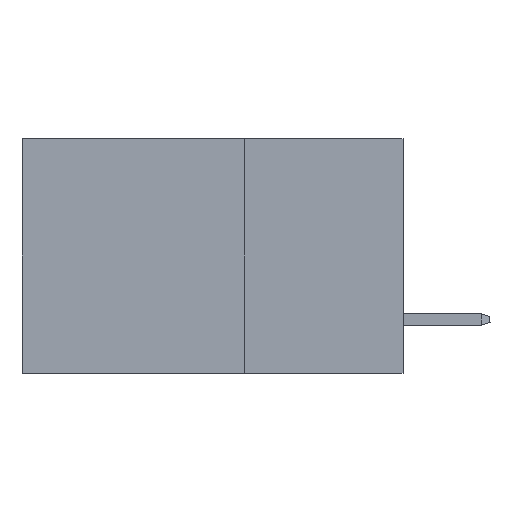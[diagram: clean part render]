
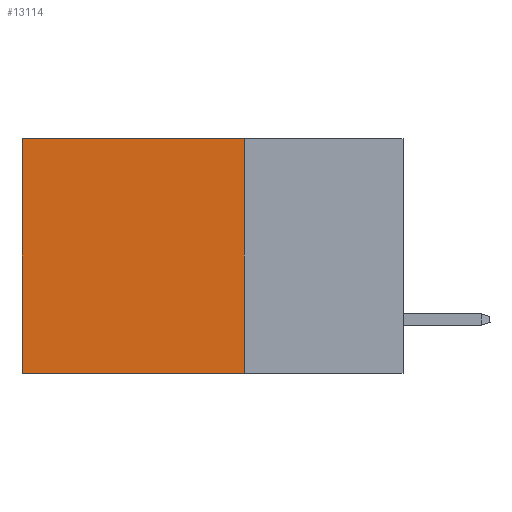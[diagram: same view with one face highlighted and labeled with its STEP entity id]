
A CAD part, left-side view. The second image highlights one B-rep face of the part: STEP entity #13114.
In plain terms, the highlighted planar face has unit normal (-1, 0, 0).
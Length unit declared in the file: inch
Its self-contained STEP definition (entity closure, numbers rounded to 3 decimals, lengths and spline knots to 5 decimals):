
#281 = EDGE_CURVE ( 'NONE', #8161, #18576, #7466, .T. ) ;
#1799 = CARTESIAN_POINT ( 'NONE',  ( 0.2875, 0.25, 0. ) ) ;
#2214 = EDGE_CURVE ( 'NONE', #22995, #3551, #21140, .T. ) ;
#2503 = CARTESIAN_POINT ( 'NONE',  ( 0.2875, 0.6, 0. ) ) ;
#2997 = EDGE_LOOP ( 'NONE', ( #9838, #13088, #6415, #18255 ) ) ;
#3185 = LINE ( 'NONE', #12892, #14481 ) ;
#3551 = VERTEX_POINT ( 'NONE', #19859 ) ;
#3918 = DIRECTION ( 'NONE',  ( 0., 1., 0. ) ) ;
#6327 = CARTESIAN_POINT ( 'NONE',  ( 0.2875, 0.6, 0. ) ) ;
#6415 = ORIENTED_EDGE ( 'NONE', *, *, #8126, .F. ) ;
#7466 = LINE ( 'NONE', #1799, #23262 ) ;
#8126 = EDGE_CURVE ( 'NONE', #8161, #22995, #3185, .T. ) ;
#8161 = VERTEX_POINT ( 'NONE', #15132 ) ;
#9838 = ORIENTED_EDGE ( 'NONE', *, *, #12506, .T. ) ;
#10534 = FACE_OUTER_BOUND ( 'NONE', #2997, .T. ) ;
#12418 = DIRECTION ( 'NONE',  ( 0., 0., -1. ) ) ;
#12506 = EDGE_CURVE ( 'NONE', #18576, #3551, #17708, .T. ) ;
#12892 = CARTESIAN_POINT ( 'NONE',  ( 0.2875, 0.25, 0. ) ) ;
#13088 = ORIENTED_EDGE ( 'NONE', *, *, #2214, .F. ) ;
#13114 = ADVANCED_FACE ( 'NONE', ( #10534 ), #18291, .F. ) ;
#13362 = CARTESIAN_POINT ( 'NONE',  ( 0.2875, 0.25, -0.37 ) ) ;
#14481 = VECTOR ( 'NONE', #20529, 39.37008 ) ;
#15132 = CARTESIAN_POINT ( 'NONE',  ( 0.2875, 0.25, 0. ) ) ;
#15911 = VECTOR ( 'NONE', #3918, 39.37008 ) ;
#16674 = CARTESIAN_POINT ( 'NONE',  ( 0.2875, 0.25, -0.37 ) ) ;
#17708 = LINE ( 'NONE', #2503, #18965 ) ;
#17952 = DIRECTION ( 'NONE',  ( 0., 0., -1. ) ) ;
#18255 = ORIENTED_EDGE ( 'NONE', *, *, #281, .T. ) ;
#18291 = PLANE ( 'NONE',  #18571 ) ;
#18571 = AXIS2_PLACEMENT_3D ( 'NONE', #22063, #24309, #12418 ) ;
#18576 = VERTEX_POINT ( 'NONE', #6327 ) ;
#18965 = VECTOR ( 'NONE', #17952, 39.37008 ) ;
#19859 = CARTESIAN_POINT ( 'NONE',  ( 0.2875, 0.6, -0.37 ) ) ;
#20529 = DIRECTION ( 'NONE',  ( 0., 0., -1. ) ) ;
#21140 = LINE ( 'NONE', #13362, #15911 ) ;
#22063 = CARTESIAN_POINT ( 'NONE',  ( 0.2875, 0.25, 0. ) ) ;
#22296 = DIRECTION ( 'NONE',  ( 0., 1., 0. ) ) ;
#22995 = VERTEX_POINT ( 'NONE', #16674 ) ;
#23262 = VECTOR ( 'NONE', #22296, 39.37008 ) ;
#24309 = DIRECTION ( 'NONE',  ( 1., 0., 0. ) ) ;
